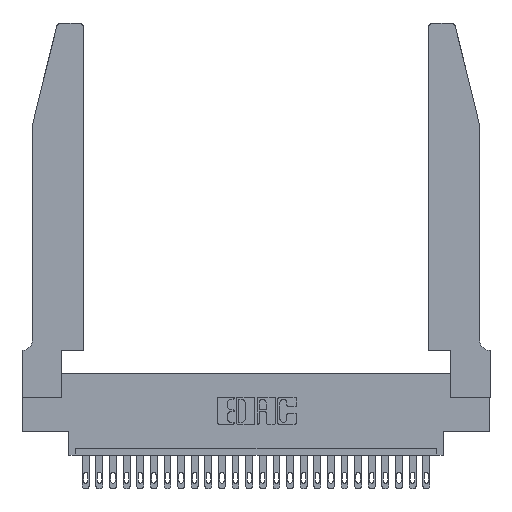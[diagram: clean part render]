
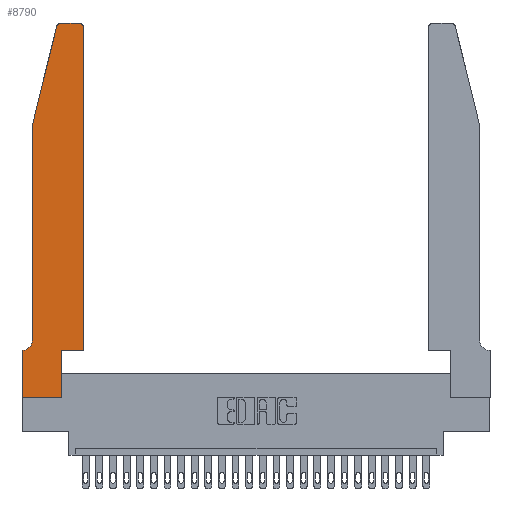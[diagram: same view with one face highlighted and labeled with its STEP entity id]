
A CAD part, top view. The second image highlights one B-rep face of the part: STEP entity #8790.
In plain terms, the highlighted planar face has unit normal (0, 0, 1).
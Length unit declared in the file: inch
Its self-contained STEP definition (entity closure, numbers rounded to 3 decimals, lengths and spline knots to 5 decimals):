
#233 = ORIENTED_EDGE ( 'NONE', *, *, #8981, .T. ) ;
#343 = CARTESIAN_POINT ( 'NONE',  ( 0.0055, 0.42, 0.37 ) ) ;
#556 = EDGE_CURVE ( 'NONE', #24808, #3152, #15498, .T. ) ;
#652 = ORIENTED_EDGE ( 'NONE', *, *, #5531, .T. ) ;
#1970 = VECTOR ( 'NONE', #24268, 39.37008 ) ;
#2553 = DIRECTION ( 'NONE',  ( 0., 0., 1. ) ) ;
#2648 = LINE ( 'NONE', #13594, #1970 ) ;
#2867 = LINE ( 'NONE', #23807, #15021 ) ;
#3053 = CARTESIAN_POINT ( 'NONE',  ( 0.2605, 2.75, 0.37 ) ) ;
#3152 = VERTEX_POINT ( 'NONE', #7962 ) ;
#3318 = EDGE_CURVE ( 'NONE', #7608, #4110, #2648, .T. ) ;
#3407 = LINE ( 'NONE', #11565, #17775 ) ;
#3593 = AXIS2_PLACEMENT_3D ( 'NONE', #343, #8913, #4778 ) ;
#4110 = VERTEX_POINT ( 'NONE', #11619 ) ;
#4381 = ORIENTED_EDGE ( 'NONE', *, *, #556, .T. ) ;
#4475 = EDGE_CURVE ( 'NONE', #4110, #21924, #25302, .T. ) ;
#4608 = VECTOR ( 'NONE', #6775, 39.37008 ) ;
#4709 = PLANE ( 'NONE',  #4903 ) ;
#4778 = DIRECTION ( 'NONE',  ( -1., 0., 0. ) ) ;
#4788 = DIRECTION ( 'NONE',  ( -1., 0., 0. ) ) ;
#4903 = AXIS2_PLACEMENT_3D ( 'NONE', #10729, #2553, #22932 ) ;
#5154 = CIRCLE ( 'NONE', #3593, 0.07 ) ;
#5385 = DIRECTION ( 'NONE',  ( 0., -1., 0. ) ) ;
#5531 = EDGE_CURVE ( 'NONE', #9356, #22133, #20146, .T. ) ;
#5877 = VERTEX_POINT ( 'NONE', #13572 ) ;
#6138 = CARTESIAN_POINT ( 'NONE',  ( 0.4205, 2.72, 0.37 ) ) ;
#6602 = CARTESIAN_POINT ( 'NONE',  ( 0., 0., 0.37 ) ) ;
#6775 = DIRECTION ( 'NONE',  ( 1., 0., 0. ) ) ;
#7020 = ORIENTED_EDGE ( 'NONE', *, *, #4475, .T. ) ;
#7266 = ORIENTED_EDGE ( 'NONE', *, *, #20487, .T. ) ;
#7307 = LINE ( 'NONE', #11617, #25848 ) ;
#7463 = ORIENTED_EDGE ( 'NONE', *, *, #12466, .T. ) ;
#7608 = VERTEX_POINT ( 'NONE', #17732 ) ;
#7896 = ORIENTED_EDGE ( 'NONE', *, *, #14341, .T. ) ;
#7962 = CARTESIAN_POINT ( 'NONE',  ( 0., 0.35, 0.37 ) ) ;
#8179 = CARTESIAN_POINT ( 'NONE',  ( 0.2865, 0.35, 0.37 ) ) ;
#8206 = DIRECTION ( 'NONE',  ( 1., 0., 0. ) ) ;
#8527 = EDGE_CURVE ( 'NONE', #18445, #18793, #7307, .T. ) ;
#8790 = ADVANCED_FACE ( 'NONE', ( #13972 ), #4709, .T. ) ;
#8913 = DIRECTION ( 'NONE',  ( 0., 0., -1. ) ) ;
#8981 = EDGE_CURVE ( 'NONE', #5877, #18445, #3407, .T. ) ;
#9356 = VERTEX_POINT ( 'NONE', #23171 ) ;
#9476 = DIRECTION ( 'NONE',  ( 1., 0., 0. ) ) ;
#9632 = DIRECTION ( 'NONE',  ( 1., 0., 0. ) ) ;
#9645 = VECTOR ( 'NONE', #14745, 39.37008 ) ;
#10689 = ORIENTED_EDGE ( 'NONE', *, *, #16928, .T. ) ;
#10704 = CARTESIAN_POINT ( 'NONE',  ( 0., 0., 0.37 ) ) ;
#10729 = CARTESIAN_POINT ( 'NONE',  ( 0., 0.35, 0.37 ) ) ;
#11482 = CARTESIAN_POINT ( 'NONE',  ( 0., 0., 0.37 ) ) ;
#11565 = CARTESIAN_POINT ( 'NONE',  ( 0.2865, 0.35, 0.37 ) ) ;
#11617 = CARTESIAN_POINT ( 'NONE',  ( 0.4505, 0.35, 0.37 ) ) ;
#11619 = CARTESIAN_POINT ( 'NONE',  ( 0.0755, 2., 0.37 ) ) ;
#12119 = CARTESIAN_POINT ( 'NONE',  ( 0.0755, 0.35, 0.37 ) ) ;
#12266 = AXIS2_PLACEMENT_3D ( 'NONE', #26317, #17705, #9632 ) ;
#12466 = EDGE_CURVE ( 'NONE', #21924, #24808, #5154, .T. ) ;
#12559 = VERTEX_POINT ( 'NONE', #10704 ) ;
#12944 = CARTESIAN_POINT ( 'NONE',  ( 0.284, 2.75, 0.37 ) ) ;
#13572 = CARTESIAN_POINT ( 'NONE',  ( 0.2865, 0., 0.37 ) ) ;
#13594 = CARTESIAN_POINT ( 'NONE',  ( 0.0755, 2., 0.37 ) ) ;
#13596 = DIRECTION ( 'NONE',  ( 0., 1., 0. ) ) ;
#13787 = EDGE_CURVE ( 'NONE', #18793, #9356, #2867, .T. ) ;
#13972 = FACE_OUTER_BOUND ( 'NONE', #24717, .T. ) ;
#14065 = ORIENTED_EDGE ( 'NONE', *, *, #13787, .T. ) ;
#14318 = CARTESIAN_POINT ( 'NONE',  ( 0.0055, 0.35, 0.37 ) ) ;
#14341 = EDGE_CURVE ( 'NONE', #22133, #21051, #20088, .T. ) ;
#14659 = VECTOR ( 'NONE', #19260, 39.37008 ) ;
#14745 = DIRECTION ( 'NONE',  ( 0., -1., 0. ) ) ;
#15021 = VECTOR ( 'NONE', #15571, 39.37008 ) ;
#15498 = LINE ( 'NONE', #12119, #22878 ) ;
#15571 = DIRECTION ( 'NONE',  ( 0., 1., 0. ) ) ;
#15964 = CARTESIAN_POINT ( 'NONE',  ( 0.0755, 0.42, 0.37 ) ) ;
#16928 = EDGE_CURVE ( 'NONE', #21051, #7608, #17532, .T. ) ;
#17532 = CIRCLE ( 'NONE', #12266, 0.03 ) ;
#17705 = DIRECTION ( 'NONE',  ( 0., 0., 1. ) ) ;
#17732 = CARTESIAN_POINT ( 'NONE',  ( 0.25487, 2.72718, 0.37 ) ) ;
#17775 = VECTOR ( 'NONE', #13596, 39.37008 ) ;
#18445 = VERTEX_POINT ( 'NONE', #8179 ) ;
#18526 = AXIS2_PLACEMENT_3D ( 'NONE', #6138, #20425, #8206 ) ;
#18793 = VERTEX_POINT ( 'NONE', #26048 ) ;
#18855 = CARTESIAN_POINT ( 'NONE',  ( 0.0755, 2., 0.37 ) ) ;
#18954 = VECTOR ( 'NONE', #5385, 39.37008 ) ;
#19260 = DIRECTION ( 'NONE',  ( -1., 0., 0. ) ) ;
#19266 = ORIENTED_EDGE ( 'NONE', *, *, #8527, .T. ) ;
#19608 = EDGE_CURVE ( 'NONE', #12559, #5877, #22485, .T. ) ;
#20088 = LINE ( 'NONE', #3053, #14659 ) ;
#20146 = CIRCLE ( 'NONE', #18526, 0.03 ) ;
#20425 = DIRECTION ( 'NONE',  ( 0., 0., 1. ) ) ;
#20487 = EDGE_CURVE ( 'NONE', #3152, #12559, #24367, .T. ) ;
#21051 = VERTEX_POINT ( 'NONE', #12944 ) ;
#21924 = VERTEX_POINT ( 'NONE', #15964 ) ;
#22133 = VERTEX_POINT ( 'NONE', #24744 ) ;
#22485 = LINE ( 'NONE', #6602, #4608 ) ;
#22878 = VECTOR ( 'NONE', #4788, 39.37008 ) ;
#22932 = DIRECTION ( 'NONE',  ( 1., 0., 0. ) ) ;
#23171 = CARTESIAN_POINT ( 'NONE',  ( 0.4505, 2.72, 0.37 ) ) ;
#23292 = ORIENTED_EDGE ( 'NONE', *, *, #3318, .T. ) ;
#23807 = CARTESIAN_POINT ( 'NONE',  ( 0.4505, 0.35, 0.37 ) ) ;
#24268 = DIRECTION ( 'NONE',  ( -0.239, -0.971, 0. ) ) ;
#24367 = LINE ( 'NONE', #11482, #18954 ) ;
#24717 = EDGE_LOOP ( 'NONE', ( #7896, #10689, #23292, #7020, #7463, #4381, #7266, #25303, #233, #19266, #14065, #652 ) ) ;
#24744 = CARTESIAN_POINT ( 'NONE',  ( 0.4205, 2.75, 0.37 ) ) ;
#24808 = VERTEX_POINT ( 'NONE', #14318 ) ;
#25302 = LINE ( 'NONE', #18855, #9645 ) ;
#25303 = ORIENTED_EDGE ( 'NONE', *, *, #19608, .T. ) ;
#25848 = VECTOR ( 'NONE', #9476, 39.37008 ) ;
#26048 = CARTESIAN_POINT ( 'NONE',  ( 0.4505, 0.35, 0.37 ) ) ;
#26317 = CARTESIAN_POINT ( 'NONE',  ( 0.284, 2.72, 0.37 ) ) ;
